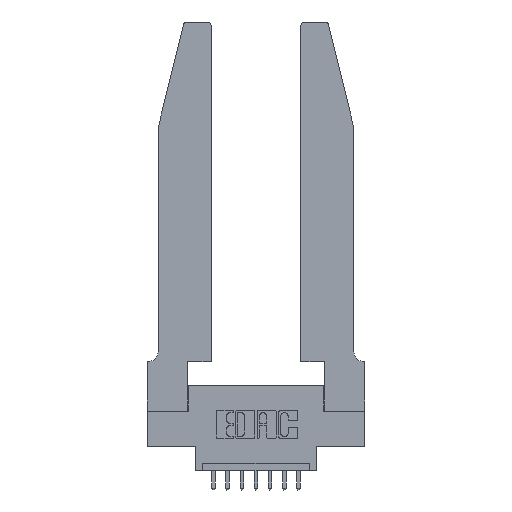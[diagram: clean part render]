
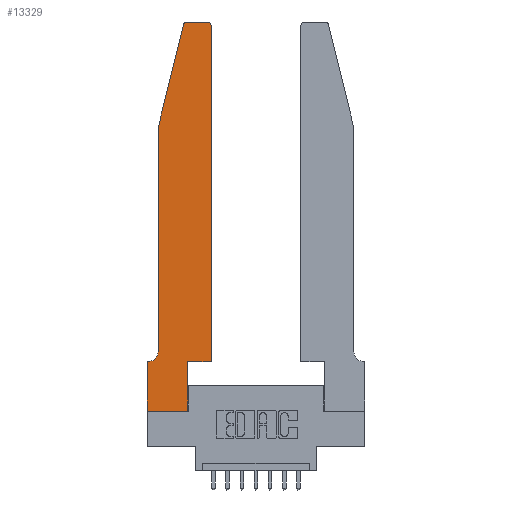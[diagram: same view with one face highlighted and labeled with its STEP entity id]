
A CAD part, top view. The second image highlights one B-rep face of the part: STEP entity #13329.
In plain terms, the highlighted planar face has unit normal (0, 0, 1).
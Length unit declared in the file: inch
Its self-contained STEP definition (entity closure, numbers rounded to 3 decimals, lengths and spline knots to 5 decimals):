
#44 = DIRECTION ( 'NONE',  ( 0., 1., 0. ) ) ;
#272 = LINE ( 'NONE', #6876, #4416 ) ;
#273 = DIRECTION ( 'NONE',  ( 0., 0., 1. ) ) ;
#598 = CARTESIAN_POINT ( 'NONE',  ( 0.0755, 2., 0.37 ) ) ;
#633 = ORIENTED_EDGE ( 'NONE', *, *, #9116, .T. ) ;
#655 = CARTESIAN_POINT ( 'NONE',  ( 0., 0., 0.37 ) ) ;
#781 = CIRCLE ( 'NONE', #5284, 0.07 ) ;
#983 = AXIS2_PLACEMENT_3D ( 'NONE', #9573, #273, #10624 ) ;
#991 = DIRECTION ( 'NONE',  ( 0., -1., 0. ) ) ;
#1045 = CARTESIAN_POINT ( 'NONE',  ( 0.4505, 0.35, 0.37 ) ) ;
#1054 = EDGE_CURVE ( 'NONE', #12914, #8360, #13611, .T. ) ;
#1060 = DIRECTION ( 'NONE',  ( -1., 0., 0. ) ) ;
#1226 = VECTOR ( 'NONE', #11090, 39.37008 ) ;
#1296 = CARTESIAN_POINT ( 'NONE',  ( 0., 0., 0.37 ) ) ;
#1704 = VERTEX_POINT ( 'NONE', #5812 ) ;
#1735 = VECTOR ( 'NONE', #6888, 39.37008 ) ;
#1955 = LINE ( 'NONE', #14688, #1226 ) ;
#2029 = VECTOR ( 'NONE', #7997, 39.37008 ) ;
#2043 = DIRECTION ( 'NONE',  ( 1., 0., 0. ) ) ;
#2713 = ORIENTED_EDGE ( 'NONE', *, *, #11629, .T. ) ;
#2857 = ORIENTED_EDGE ( 'NONE', *, *, #12994, .T. ) ;
#3047 = VECTOR ( 'NONE', #1060, 39.37008 ) ;
#3588 = FACE_OUTER_BOUND ( 'NONE', #4161, .T. ) ;
#4161 = EDGE_LOOP ( 'NONE', ( #13126, #8359, #2713, #4998, #12429, #11203, #633, #2857, #9856, #9784, #9869, #5734 ) ) ;
#4350 = VERTEX_POINT ( 'NONE', #14373 ) ;
#4416 = VECTOR ( 'NONE', #44, 39.37008 ) ;
#4998 = ORIENTED_EDGE ( 'NONE', *, *, #9220, .T. ) ;
#5265 = CARTESIAN_POINT ( 'NONE',  ( 0.4505, 2.72, 0.37 ) ) ;
#5284 = AXIS2_PLACEMENT_3D ( 'NONE', #8446, #12027, #7327 ) ;
#5513 = VERTEX_POINT ( 'NONE', #8761 ) ;
#5640 = LINE ( 'NONE', #5712, #2029 ) ;
#5712 = CARTESIAN_POINT ( 'NONE',  ( 0.0755, 2., 0.37 ) ) ;
#5734 = ORIENTED_EDGE ( 'NONE', *, *, #1054, .T. ) ;
#5812 = CARTESIAN_POINT ( 'NONE',  ( 0.0055, 0.35, 0.37 ) ) ;
#6006 = DIRECTION ( 'NONE',  ( 1., 0., 0. ) ) ;
#6569 = VERTEX_POINT ( 'NONE', #8626 ) ;
#6613 = VERTEX_POINT ( 'NONE', #11956 ) ;
#6849 = VECTOR ( 'NONE', #13413, 39.37008 ) ;
#6876 = CARTESIAN_POINT ( 'NONE',  ( 0.4505, 0.35, 0.37 ) ) ;
#6888 = DIRECTION ( 'NONE',  ( -1., 0., 0. ) ) ;
#7088 = DIRECTION ( 'NONE',  ( 1., 0., 0. ) ) ;
#7250 = CIRCLE ( 'NONE', #8554, 0.03 ) ;
#7327 = DIRECTION ( 'NONE',  ( -1., 0., 0. ) ) ;
#7542 = VECTOR ( 'NONE', #8755, 39.37008 ) ;
#7600 = VECTOR ( 'NONE', #991, 39.37008 ) ;
#7631 = CARTESIAN_POINT ( 'NONE',  ( 0.2865, 0.35, 0.37 ) ) ;
#7746 = EDGE_CURVE ( 'NONE', #5513, #12914, #272, .T. ) ;
#7775 = CARTESIAN_POINT ( 'NONE',  ( 0.2605, 2.75, 0.37 ) ) ;
#7795 = VECTOR ( 'NONE', #2043, 39.37008 ) ;
#7918 = LINE ( 'NONE', #9223, #6849 ) ;
#7997 = DIRECTION ( 'NONE',  ( 0., -1., 0. ) ) ;
#8240 = EDGE_CURVE ( 'NONE', #14593, #5513, #9435, .T. ) ;
#8293 = LINE ( 'NONE', #14576, #7542 ) ;
#8351 = CARTESIAN_POINT ( 'NONE',  ( 0.4205, 2.72, 0.37 ) ) ;
#8359 = ORIENTED_EDGE ( 'NONE', *, *, #8828, .T. ) ;
#8360 = VERTEX_POINT ( 'NONE', #13997 ) ;
#8407 = PLANE ( 'NONE',  #983 ) ;
#8446 = CARTESIAN_POINT ( 'NONE',  ( 0.0055, 0.42, 0.37 ) ) ;
#8554 = AXIS2_PLACEMENT_3D ( 'NONE', #10506, #9461, #7088 ) ;
#8626 = CARTESIAN_POINT ( 'NONE',  ( 0.2865, 0., 0.37 ) ) ;
#8755 = DIRECTION ( 'NONE',  ( 0., 1., 0. ) ) ;
#8761 = CARTESIAN_POINT ( 'NONE',  ( 0.4505, 0.35, 0.37 ) ) ;
#8769 = VERTEX_POINT ( 'NONE', #9118 ) ;
#8816 = VERTEX_POINT ( 'NONE', #12887 ) ;
#8828 = EDGE_CURVE ( 'NONE', #8769, #8816, #7250, .T. ) ;
#8936 = EDGE_CURVE ( 'NONE', #6613, #1704, #781, .T. ) ;
#9116 = EDGE_CURVE ( 'NONE', #4350, #9682, #14255, .T. ) ;
#9118 = CARTESIAN_POINT ( 'NONE',  ( 0.284, 2.75, 0.37 ) ) ;
#9220 = EDGE_CURVE ( 'NONE', #14042, #6613, #5640, .T. ) ;
#9223 = CARTESIAN_POINT ( 'NONE',  ( 0.0755, 2., 0.37 ) ) ;
#9435 = LINE ( 'NONE', #1045, #7795 ) ;
#9461 = DIRECTION ( 'NONE',  ( 0., 0., 1. ) ) ;
#9573 = CARTESIAN_POINT ( 'NONE',  ( 0., 0.35, 0.37 ) ) ;
#9682 = VERTEX_POINT ( 'NONE', #1296 ) ;
#9784 = ORIENTED_EDGE ( 'NONE', *, *, #8240, .T. ) ;
#9856 = ORIENTED_EDGE ( 'NONE', *, *, #10374, .T. ) ;
#9869 = ORIENTED_EDGE ( 'NONE', *, *, #7746, .T. ) ;
#10374 = EDGE_CURVE ( 'NONE', #6569, #14593, #8293, .T. ) ;
#10506 = CARTESIAN_POINT ( 'NONE',  ( 0.284, 2.72, 0.37 ) ) ;
#10552 = EDGE_CURVE ( 'NONE', #8360, #8769, #12766, .T. ) ;
#10624 = DIRECTION ( 'NONE',  ( 1., 0., 0. ) ) ;
#11090 = DIRECTION ( 'NONE',  ( 1., 0., 0. ) ) ;
#11203 = ORIENTED_EDGE ( 'NONE', *, *, #14647, .T. ) ;
#11390 = AXIS2_PLACEMENT_3D ( 'NONE', #8351, #11697, #6006 ) ;
#11629 = EDGE_CURVE ( 'NONE', #8816, #14042, #7918, .T. ) ;
#11697 = DIRECTION ( 'NONE',  ( 0., 0., 1. ) ) ;
#11956 = CARTESIAN_POINT ( 'NONE',  ( 0.0755, 0.42, 0.37 ) ) ;
#12027 = DIRECTION ( 'NONE',  ( 0., 0., -1. ) ) ;
#12429 = ORIENTED_EDGE ( 'NONE', *, *, #8936, .T. ) ;
#12703 = LINE ( 'NONE', #13892, #1735 ) ;
#12766 = LINE ( 'NONE', #7775, #3047 ) ;
#12887 = CARTESIAN_POINT ( 'NONE',  ( 0.25487, 2.72718, 0.37 ) ) ;
#12914 = VERTEX_POINT ( 'NONE', #5265 ) ;
#12994 = EDGE_CURVE ( 'NONE', #9682, #6569, #1955, .T. ) ;
#13126 = ORIENTED_EDGE ( 'NONE', *, *, #10552, .T. ) ;
#13329 = ADVANCED_FACE ( 'NONE', ( #3588 ), #8407, .T. ) ;
#13413 = DIRECTION ( 'NONE',  ( -0.239, -0.971, 0. ) ) ;
#13611 = CIRCLE ( 'NONE', #11390, 0.03 ) ;
#13892 = CARTESIAN_POINT ( 'NONE',  ( 0.0755, 0.35, 0.37 ) ) ;
#13997 = CARTESIAN_POINT ( 'NONE',  ( 0.4205, 2.75, 0.37 ) ) ;
#14042 = VERTEX_POINT ( 'NONE', #598 ) ;
#14255 = LINE ( 'NONE', #655, #7600 ) ;
#14373 = CARTESIAN_POINT ( 'NONE',  ( 0., 0.35, 0.37 ) ) ;
#14576 = CARTESIAN_POINT ( 'NONE',  ( 0.2865, 0.35, 0.37 ) ) ;
#14593 = VERTEX_POINT ( 'NONE', #7631 ) ;
#14647 = EDGE_CURVE ( 'NONE', #1704, #4350, #12703, .T. ) ;
#14688 = CARTESIAN_POINT ( 'NONE',  ( 0., 0., 0.37 ) ) ;
